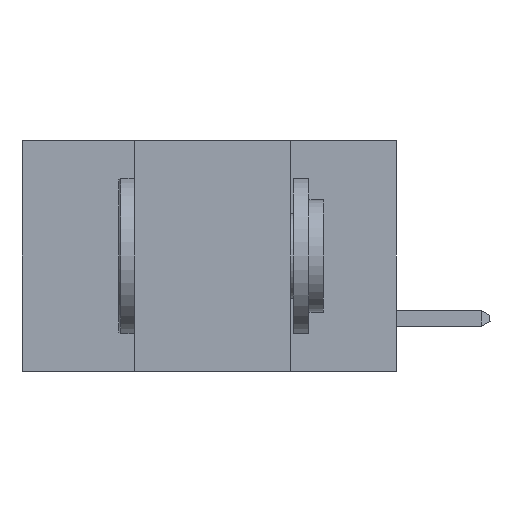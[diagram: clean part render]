
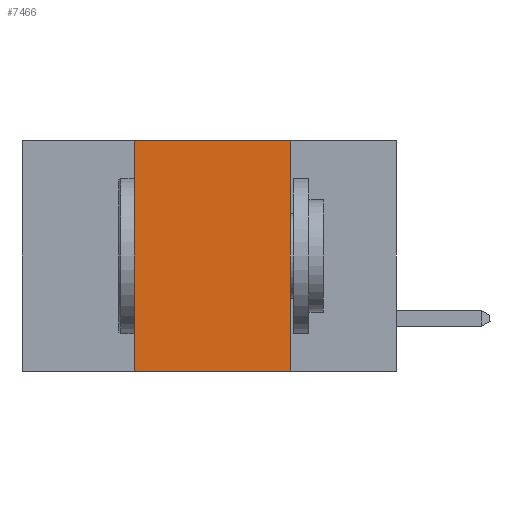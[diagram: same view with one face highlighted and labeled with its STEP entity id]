
A CAD part, left-side view. The second image highlights one B-rep face of the part: STEP entity #7466.
In plain terms, the highlighted planar face has unit normal (-1, 0, 0).
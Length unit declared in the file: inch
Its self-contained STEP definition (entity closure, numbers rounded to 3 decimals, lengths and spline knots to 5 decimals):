
#762 = CARTESIAN_POINT ( 'NONE',  ( 0., 0.6, -0.37 ) ) ;
#1199 = DIRECTION ( 'NONE',  ( 0., 0., -1. ) ) ;
#2695 = FACE_OUTER_BOUND ( 'NONE', #13368, .T. ) ;
#3528 = CARTESIAN_POINT ( 'NONE',  ( 0., 0.42, 0. ) ) ;
#4283 = DIRECTION ( 'NONE',  ( 0., 0., -1. ) ) ;
#4321 = DIRECTION ( 'NONE',  ( 1., 0., 0. ) ) ;
#4354 = CARTESIAN_POINT ( 'NONE',  ( 0., 0.6, 0. ) ) ;
#4503 = PLANE ( 'NONE',  #4920 ) ;
#4920 = AXIS2_PLACEMENT_3D ( 'NONE', #4354, #4321, #4283 ) ;
#5145 = EDGE_CURVE ( 'NONE', #5542, #30758, #28484, .T. ) ;
#5542 = VERTEX_POINT ( 'NONE', #3528 ) ;
#6431 = VERTEX_POINT ( 'NONE', #20700 ) ;
#7466 = ADVANCED_FACE ( 'NONE', ( #2695 ), #4503, .F. ) ;
#7777 = DIRECTION ( 'NONE',  ( 0., 0., 1. ) ) ;
#7969 = EDGE_CURVE ( 'NONE', #30758, #17334, #27856, .T. ) ;
#11411 = CARTESIAN_POINT ( 'NONE',  ( 0., 0.17, 0. ) ) ;
#12872 = CARTESIAN_POINT ( 'NONE',  ( 0., 0.42, 0. ) ) ;
#13368 = EDGE_LOOP ( 'NONE', ( #16613, #17493, #19241, #19712 ) ) ;
#14536 = VECTOR ( 'NONE', #1199, 39.37008 ) ;
#15940 = VECTOR ( 'NONE', #19235, 39.37008 ) ;
#16613 = ORIENTED_EDGE ( 'NONE', *, *, #7969, .F. ) ;
#17291 = CARTESIAN_POINT ( 'NONE',  ( 0., 0.17, -0.37 ) ) ;
#17334 = VERTEX_POINT ( 'NONE', #17291 ) ;
#17493 = ORIENTED_EDGE ( 'NONE', *, *, #5145, .F. ) ;
#19235 = DIRECTION ( 'NONE',  ( 0., -1., 0. ) ) ;
#19241 = ORIENTED_EDGE ( 'NONE', *, *, #20402, .F. ) ;
#19338 = CARTESIAN_POINT ( 'NONE',  ( 0., 0.6, 0. ) ) ;
#19712 = ORIENTED_EDGE ( 'NONE', *, *, #26061, .T. ) ;
#20052 = CARTESIAN_POINT ( 'NONE',  ( 0., 0.17, 0. ) ) ;
#20402 = EDGE_CURVE ( 'NONE', #6431, #5542, #24682, .T. ) ;
#20700 = CARTESIAN_POINT ( 'NONE',  ( 0., 0.42, -0.37 ) ) ;
#23899 = VECTOR ( 'NONE', #7777, 39.37008 ) ;
#24682 = LINE ( 'NONE', #12872, #23899 ) ;
#24844 = VECTOR ( 'NONE', #28540, 39.37008 ) ;
#26061 = EDGE_CURVE ( 'NONE', #6431, #17334, #31551, .T. ) ;
#27856 = LINE ( 'NONE', #11411, #14536 ) ;
#28484 = LINE ( 'NONE', #19338, #15940 ) ;
#28540 = DIRECTION ( 'NONE',  ( 0., -1., 0. ) ) ;
#30758 = VERTEX_POINT ( 'NONE', #20052 ) ;
#31551 = LINE ( 'NONE', #762, #24844 ) ;
